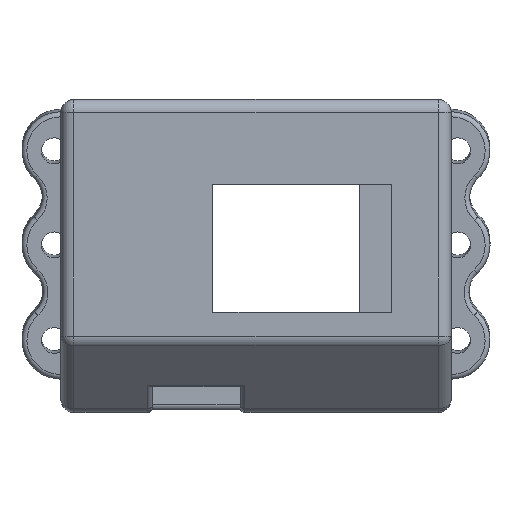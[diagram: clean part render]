
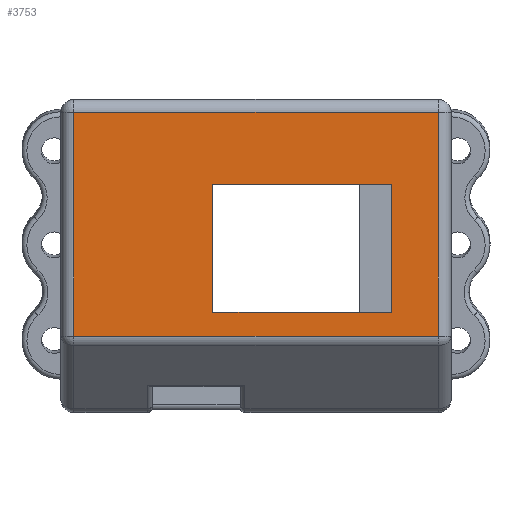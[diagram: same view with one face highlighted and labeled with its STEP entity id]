
A CAD part, top view. The second image highlights one B-rep face of the part: STEP entity #3753.
In plain terms, the highlighted planar face has unit normal (0, 0, 1).
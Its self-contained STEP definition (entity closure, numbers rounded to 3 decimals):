
#246=FACE_BOUND('',#813,.T.);
#579=FACE_OUTER_BOUND('',#812,.T.);
#812=EDGE_LOOP('',(#2701,#2702,#2703,#2704));
#813=EDGE_LOOP('',(#2705,#2706,#2707,#2708));
#1084=LINE('',#5765,#1333);
#1165=LINE('',#5994,#1414);
#1167=LINE('',#5999,#1416);
#1168=LINE('',#6001,#1417);
#1169=LINE('',#6003,#1418);
#1170=LINE('',#6004,#1419);
#1171=LINE('',#6005,#1420);
#1172=LINE('',#6006,#1421);
#1333=VECTOR('',#4516,10.);
#1414=VECTOR('',#4691,10.);
#1416=VECTOR('',#4695,10.);
#1417=VECTOR('',#4696,10.);
#1418=VECTOR('',#4697,10.);
#1419=VECTOR('',#4698,10.);
#1420=VECTOR('',#4699,10.);
#1421=VECTOR('',#4700,10.);
#1588=VERTEX_POINT('',#5762);
#1589=VERTEX_POINT('',#5764);
#1673=VERTEX_POINT('',#5991);
#1674=VERTEX_POINT('',#5993);
#1675=VERTEX_POINT('',#5997);
#1676=VERTEX_POINT('',#5998);
#1677=VERTEX_POINT('',#6000);
#1678=VERTEX_POINT('',#6002);
#1958=EDGE_CURVE('',#1589,#1588,#1084,.T.);
#2067=EDGE_CURVE('',#1674,#1673,#1165,.T.);
#2069=EDGE_CURVE('',#1675,#1676,#1167,.T.);
#2070=EDGE_CURVE('',#1677,#1675,#1168,.T.);
#2071=EDGE_CURVE('',#1678,#1677,#1169,.T.);
#2072=EDGE_CURVE('',#1676,#1678,#1170,.T.);
#2073=EDGE_CURVE('',#1588,#1674,#1171,.T.);
#2074=EDGE_CURVE('',#1673,#1589,#1172,.T.);
#2701=ORIENTED_EDGE('',*,*,#2069,.F.);
#2702=ORIENTED_EDGE('',*,*,#2070,.F.);
#2703=ORIENTED_EDGE('',*,*,#2071,.F.);
#2704=ORIENTED_EDGE('',*,*,#2072,.F.);
#2705=ORIENTED_EDGE('',*,*,#2073,.T.);
#2706=ORIENTED_EDGE('',*,*,#2067,.T.);
#2707=ORIENTED_EDGE('',*,*,#2074,.T.);
#2708=ORIENTED_EDGE('',*,*,#1958,.T.);
#3679=PLANE('',#4031);
#3753=ADVANCED_FACE('',(#579,#246),#3679,.T.);
#4031=AXIS2_PLACEMENT_3D('',#5996,#4693,#4694);
#4516=DIRECTION('',(1.,0.,0.));
#4691=DIRECTION('',(-1.,0.,0.));
#4693=DIRECTION('center_axis',(0.,0.,1.));
#4694=DIRECTION('ref_axis',(1.,0.,0.));
#4695=DIRECTION('',(-1.,0.,0.));
#4696=DIRECTION('',(0.,-1.,0.));
#4697=DIRECTION('',(1.,0.,0.));
#4698=DIRECTION('',(0.,1.,0.));
#4699=DIRECTION('',(0.,-1.,0.));
#4700=DIRECTION('',(0.,1.,0.));
#5762=CARTESIAN_POINT('',(20.956,-13.138,267.));
#5764=CARTESIAN_POINT('',(-6.656,-13.138,267.));
#5765=CARTESIAN_POINT('',(-3.328,-13.138,267.));
#5991=CARTESIAN_POINT('',(-6.656,-32.934,267.));
#5993=CARTESIAN_POINT('',(20.956,-32.934,267.));
#5994=CARTESIAN_POINT('',(10.478,-32.934,267.));
#5996=CARTESIAN_POINT('Origin',(0.,-24.313,267.));
#5997=CARTESIAN_POINT('',(28.1,-36.614,267.));
#5998=CARTESIAN_POINT('',(-28.1,-36.614,267.));
#5999=CARTESIAN_POINT('',(5.8,-36.614,267.));
#6000=CARTESIAN_POINT('',(28.1,-2.086,267.));
#6001=CARTESIAN_POINT('',(28.1,-24.313,267.));
#6002=CARTESIAN_POINT('',(-28.1,-2.086,267.));
#6003=CARTESIAN_POINT('',(8.05,-2.086,267.));
#6004=CARTESIAN_POINT('',(-28.1,-24.313,267.));
#6005=CARTESIAN_POINT('',(20.956,-18.725,267.));
#6006=CARTESIAN_POINT('',(-6.656,-28.623,267.));
